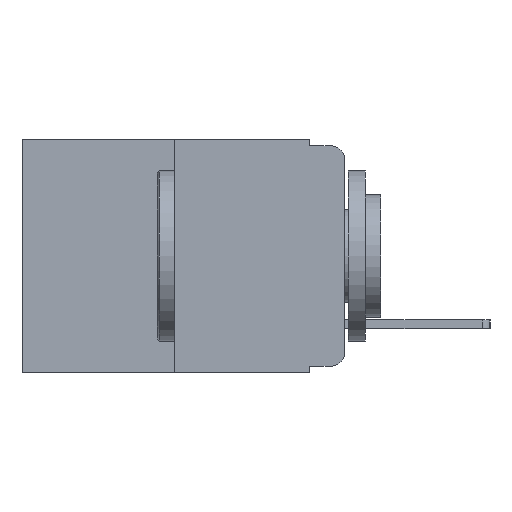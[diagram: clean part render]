
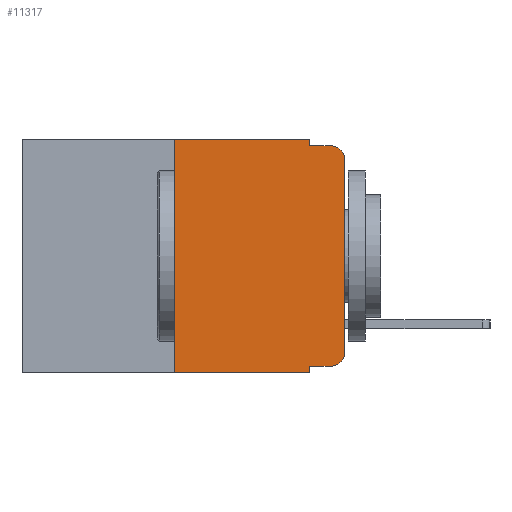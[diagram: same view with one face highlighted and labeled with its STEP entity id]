
A CAD part, left-side view. The second image highlights one B-rep face of the part: STEP entity #11317.
In plain terms, the highlighted planar face has unit normal (-1, 0, 0).
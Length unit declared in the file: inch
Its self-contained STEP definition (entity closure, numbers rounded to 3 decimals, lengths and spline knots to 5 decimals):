
#547 = VERTEX_POINT ( 'NONE', #10059 ) ;
#737 = ORIENTED_EDGE ( 'NONE', *, *, #4497, .F. ) ;
#1128 = CARTESIAN_POINT ( 'NONE',  ( 0., 0.051, -0.333 ) ) ;
#1131 = EDGE_LOOP ( 'NONE', ( #14250, #3285, #3728, #11398, #4209, #737, #8986, #12710, #16410, #16850 ) ) ;
#1167 = LINE ( 'NONE', #14059, #8487 ) ;
#1313 = VECTOR ( 'NONE', #9899, 39.37008 ) ;
#1326 = DIRECTION ( 'NONE',  ( -1., 0., 0. ) ) ;
#1375 = DIRECTION ( 'NONE',  ( 0., -1., 0. ) ) ;
#1539 = EDGE_CURVE ( 'NONE', #13473, #10609, #10692, .T. ) ;
#1725 = DIRECTION ( 'NONE',  ( 0., -1., 0. ) ) ;
#1869 = VECTOR ( 'NONE', #5631, 39.37008 ) ;
#1959 = CARTESIAN_POINT ( 'NONE',  ( 0., 0.051, 0. ) ) ;
#2432 = CARTESIAN_POINT ( 'NONE',  ( 0., 0., -0.313 ) ) ;
#2480 = PLANE ( 'NONE',  #13114 ) ;
#2526 = EDGE_CURVE ( 'NONE', #13929, #13473, #17218, .T. ) ;
#3001 = VERTEX_POINT ( 'NONE', #13475 ) ;
#3159 = CARTESIAN_POINT ( 'NONE',  ( 0., 0.051, -0.01 ) ) ;
#3285 = ORIENTED_EDGE ( 'NONE', *, *, #7440, .T. ) ;
#3363 = VERTEX_POINT ( 'NONE', #3159 ) ;
#3486 = EDGE_CURVE ( 'NONE', #13929, #14720, #17580, .T. ) ;
#3506 = VECTOR ( 'NONE', #4040, 39.37008 ) ;
#3560 = CARTESIAN_POINT ( 'NONE',  ( 0., 0.051, -0.343 ) ) ;
#3728 = ORIENTED_EDGE ( 'NONE', *, *, #6475, .F. ) ;
#4040 = DIRECTION ( 'NONE',  ( 0., 0., -1. ) ) ;
#4209 = ORIENTED_EDGE ( 'NONE', *, *, #17658, .F. ) ;
#4349 = AXIS2_PLACEMENT_3D ( 'NONE', #10022, #1326, #11437 ) ;
#4497 = EDGE_CURVE ( 'NONE', #3001, #547, #15821, .T. ) ;
#4689 = CARTESIAN_POINT ( 'NONE',  ( 0., 0.02, -0.313 ) ) ;
#4713 = DIRECTION ( 'NONE',  ( -1., 0., 0. ) ) ;
#5328 = CARTESIAN_POINT ( 'NONE',  ( 0., 0.051, 0. ) ) ;
#5495 = EDGE_CURVE ( 'NONE', #7725, #3363, #14468, .T. ) ;
#5631 = DIRECTION ( 'NONE',  ( 0., -1., 0. ) ) ;
#6475 = EDGE_CURVE ( 'NONE', #3363, #6624, #16821, .T. ) ;
#6624 = VERTEX_POINT ( 'NONE', #14592 ) ;
#6908 = CARTESIAN_POINT ( 'NONE',  ( 0., 0.473, 0. ) ) ;
#7440 = EDGE_CURVE ( 'NONE', #13709, #6624, #14388, .T. ) ;
#7725 = VERTEX_POINT ( 'NONE', #1959 ) ;
#8353 = DIRECTION ( 'NONE',  ( 0., 0., -1. ) ) ;
#8361 = VECTOR ( 'NONE', #11621, 39.37008 ) ;
#8487 = VECTOR ( 'NONE', #9868, 39.37008 ) ;
#8664 = CARTESIAN_POINT ( 'NONE',  ( 0., 0.051, -0.01 ) ) ;
#8986 = ORIENTED_EDGE ( 'NONE', *, *, #15571, .T. ) ;
#9346 = EDGE_CURVE ( 'NONE', #10609, #13709, #1167, .T. ) ;
#9736 = CARTESIAN_POINT ( 'NONE',  ( 0., 0., -0.03 ) ) ;
#9868 = DIRECTION ( 'NONE',  ( 0., 0., 1. ) ) ;
#9899 = DIRECTION ( 'NONE',  ( 0., -1., 0. ) ) ;
#10022 = CARTESIAN_POINT ( 'NONE',  ( 0., 0.02, -0.03 ) ) ;
#10059 = CARTESIAN_POINT ( 'NONE',  ( 0., 0.25, 0. ) ) ;
#10161 = VECTOR ( 'NONE', #14520, 39.37008 ) ;
#10333 = CARTESIAN_POINT ( 'NONE',  ( 0., 0.051, 0. ) ) ;
#10609 = VERTEX_POINT ( 'NONE', #2432 ) ;
#10692 = CIRCLE ( 'NONE', #17999, 0.02 ) ;
#11317 = ADVANCED_FACE ( 'NONE', ( #15199 ), #2480, .F. ) ;
#11345 = DIRECTION ( 'NONE',  ( 0., 0., -1. ) ) ;
#11398 = ORIENTED_EDGE ( 'NONE', *, *, #5495, .F. ) ;
#11437 = DIRECTION ( 'NONE',  ( 0., 0., -1. ) ) ;
#11510 = CARTESIAN_POINT ( 'NONE',  ( 0., 0.25, 0. ) ) ;
#11621 = DIRECTION ( 'NONE',  ( 0., 0., 1. ) ) ;
#12230 = VECTOR ( 'NONE', #1375, 39.37008 ) ;
#12695 = CARTESIAN_POINT ( 'NONE',  ( 0., 0.473, -0.343 ) ) ;
#12710 = ORIENTED_EDGE ( 'NONE', *, *, #3486, .F. ) ;
#12800 = LINE ( 'NONE', #16807, #1313 ) ;
#13114 = AXIS2_PLACEMENT_3D ( 'NONE', #6908, #16727, #8353 ) ;
#13327 = LINE ( 'NONE', #12695, #1869 ) ;
#13473 = VERTEX_POINT ( 'NONE', #17623 ) ;
#13475 = CARTESIAN_POINT ( 'NONE',  ( 0., 0.25, -0.343 ) ) ;
#13509 = VECTOR ( 'NONE', #1725, 39.37008 ) ;
#13709 = VERTEX_POINT ( 'NONE', #9736 ) ;
#13929 = VERTEX_POINT ( 'NONE', #17187 ) ;
#14059 = CARTESIAN_POINT ( 'NONE',  ( 0., 0., 0. ) ) ;
#14250 = ORIENTED_EDGE ( 'NONE', *, *, #9346, .T. ) ;
#14388 = CIRCLE ( 'NONE', #4349, 0.02 ) ;
#14468 = LINE ( 'NONE', #5328, #3506 ) ;
#14520 = DIRECTION ( 'NONE',  ( 0., 0., -1. ) ) ;
#14592 = CARTESIAN_POINT ( 'NONE',  ( 0., 0.02, -0.01 ) ) ;
#14720 = VERTEX_POINT ( 'NONE', #3560 ) ;
#15199 = FACE_OUTER_BOUND ( 'NONE', #1131, .T. ) ;
#15571 = EDGE_CURVE ( 'NONE', #3001, #14720, #13327, .T. ) ;
#15821 = LINE ( 'NONE', #11510, #8361 ) ;
#16410 = ORIENTED_EDGE ( 'NONE', *, *, #2526, .T. ) ;
#16727 = DIRECTION ( 'NONE',  ( 1., 0., 0. ) ) ;
#16807 = CARTESIAN_POINT ( 'NONE',  ( 0., 0.473, 0. ) ) ;
#16821 = LINE ( 'NONE', #8664, #12230 ) ;
#16850 = ORIENTED_EDGE ( 'NONE', *, *, #1539, .T. ) ;
#17187 = CARTESIAN_POINT ( 'NONE',  ( 0., 0.051, -0.333 ) ) ;
#17218 = LINE ( 'NONE', #1128, #13509 ) ;
#17580 = LINE ( 'NONE', #10333, #10161 ) ;
#17623 = CARTESIAN_POINT ( 'NONE',  ( 0., 0.02, -0.333 ) ) ;
#17658 = EDGE_CURVE ( 'NONE', #547, #7725, #12800, .T. ) ;
#17999 = AXIS2_PLACEMENT_3D ( 'NONE', #4689, #4713, #11345 ) ;
